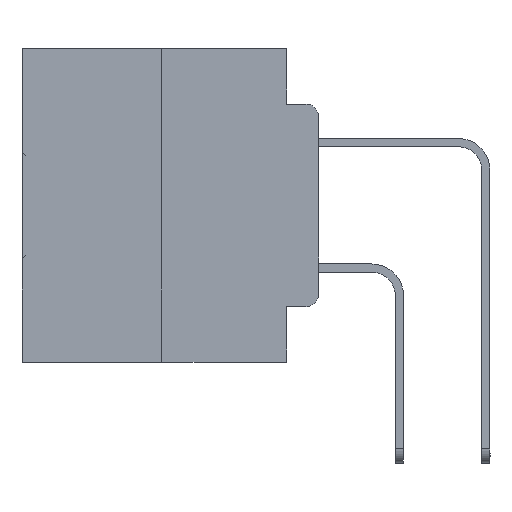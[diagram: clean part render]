
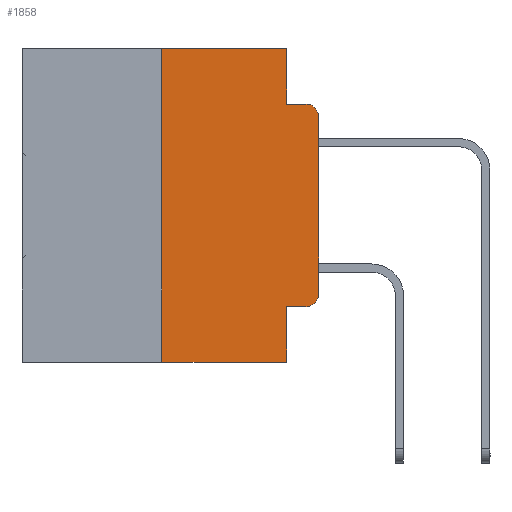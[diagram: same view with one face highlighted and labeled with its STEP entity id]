
A CAD part, left-side view. The second image highlights one B-rep face of the part: STEP entity #1858.
In plain terms, the highlighted planar face has unit normal (-1, 0, 0).
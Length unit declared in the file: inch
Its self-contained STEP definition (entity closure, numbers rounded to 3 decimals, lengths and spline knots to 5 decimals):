
#22 = CARTESIAN_POINT ( 'NONE',  ( 0., 0.25, 0. ) ) ;
#199 = ORIENTED_EDGE ( 'NONE', *, *, #5075, .F. ) ;
#231 = LINE ( 'NONE', #3575, #17360 ) ;
#294 = DIRECTION ( 'NONE',  ( -1., 0., 0. ) ) ;
#1390 = EDGE_CURVE ( 'NONE', #17032, #9484, #21260, .T. ) ;
#1604 = VECTOR ( 'NONE', #10682, 39.37008 ) ;
#1858 = ADVANCED_FACE ( 'NONE', ( #7118 ), #23116, .F. ) ;
#3144 = CARTESIAN_POINT ( 'NONE',  ( 0., 0., -0.3915 ) ) ;
#3575 = CARTESIAN_POINT ( 'NONE',  ( 0., 0., 0. ) ) ;
#3647 = AXIS2_PLACEMENT_3D ( 'NONE', #30141, #19464, #21884 ) ;
#4363 = VECTOR ( 'NONE', #18520, 39.37008 ) ;
#5075 = EDGE_CURVE ( 'NONE', #10746, #28352, #26570, .T. ) ;
#5642 = CARTESIAN_POINT ( 'NONE',  ( 0., 0.473, 0. ) ) ;
#6582 = CARTESIAN_POINT ( 'NONE',  ( 0., 0.051, -0.0885 ) ) ;
#6730 = CARTESIAN_POINT ( 'NONE',  ( 0., 0.473, 0. ) ) ;
#6943 = DIRECTION ( 'NONE',  ( 0., -1., 0. ) ) ;
#7118 = FACE_OUTER_BOUND ( 'NONE', #14256, .T. ) ;
#7145 = CARTESIAN_POINT ( 'NONE',  ( 0., 0.051, -0.5 ) ) ;
#8038 = CARTESIAN_POINT ( 'NONE',  ( 0., 0.051, 0. ) ) ;
#8712 = ORIENTED_EDGE ( 'NONE', *, *, #24335, .F. ) ;
#9397 = EDGE_CURVE ( 'NONE', #28352, #13922, #19731, .T. ) ;
#9484 = VERTEX_POINT ( 'NONE', #28569 ) ;
#10420 = CIRCLE ( 'NONE', #10743, 0.02 ) ;
#10559 = VECTOR ( 'NONE', #24782, 39.37008 ) ;
#10682 = DIRECTION ( 'NONE',  ( 0., 0., 1. ) ) ;
#10743 = AXIS2_PLACEMENT_3D ( 'NONE', #27555, #294, #19522 ) ;
#10746 = VERTEX_POINT ( 'NONE', #14887 ) ;
#10844 = CARTESIAN_POINT ( 'NONE',  ( 0., 0.25, -0.5 ) ) ;
#11346 = ORIENTED_EDGE ( 'NONE', *, *, #9397, .F. ) ;
#12129 = ORIENTED_EDGE ( 'NONE', *, *, #1390, .F. ) ;
#12223 = VECTOR ( 'NONE', #17129, 39.37008 ) ;
#13192 = ORIENTED_EDGE ( 'NONE', *, *, #17278, .T. ) ;
#13922 = VERTEX_POINT ( 'NONE', #33876 ) ;
#13999 = EDGE_CURVE ( 'NONE', #17032, #24507, #29745, .T. ) ;
#14052 = CARTESIAN_POINT ( 'NONE',  ( 0., 0.051, -0.4115 ) ) ;
#14256 = EDGE_LOOP ( 'NONE', ( #22071, #32693, #11346, #199, #30178, #12129, #21012, #8712, #13192, #14277 ) ) ;
#14277 = ORIENTED_EDGE ( 'NONE', *, *, #23934, .T. ) ;
#14463 = AXIS2_PLACEMENT_3D ( 'NONE', #6730, #34080, #25751 ) ;
#14887 = CARTESIAN_POINT ( 'NONE',  ( 0., 0.051, 0. ) ) ;
#15261 = CARTESIAN_POINT ( 'NONE',  ( 0., 0.051, 0. ) ) ;
#17032 = VERTEX_POINT ( 'NONE', #10844 ) ;
#17129 = DIRECTION ( 'NONE',  ( 0., -1., 0. ) ) ;
#17278 = EDGE_CURVE ( 'NONE', #30012, #27036, #19028, .T. ) ;
#17360 = VECTOR ( 'NONE', #19700, 39.37008 ) ;
#17816 = LINE ( 'NONE', #5642, #10559 ) ;
#18009 = DIRECTION ( 'NONE',  ( 0., 0., -1. ) ) ;
#18520 = DIRECTION ( 'NONE',  ( 0., 0., -1. ) ) ;
#18726 = CARTESIAN_POINT ( 'NONE',  ( 0., 0., -0.1085 ) ) ;
#19028 = LINE ( 'NONE', #33123, #12223 ) ;
#19464 = DIRECTION ( 'NONE',  ( -1., 0., 0. ) ) ;
#19522 = DIRECTION ( 'NONE',  ( 0., 0., -1. ) ) ;
#19700 = DIRECTION ( 'NONE',  ( 0., 0., 1. ) ) ;
#19731 = LINE ( 'NONE', #6582, #27869 ) ;
#20328 = VERTEX_POINT ( 'NONE', #3144 ) ;
#20470 = DIRECTION ( 'NONE',  ( 0., -1., 0. ) ) ;
#21012 = ORIENTED_EDGE ( 'NONE', *, *, #13999, .T. ) ;
#21260 = LINE ( 'NONE', #22, #1604 ) ;
#21812 = VERTEX_POINT ( 'NONE', #18726 ) ;
#21884 = DIRECTION ( 'NONE',  ( 0., 0., -1. ) ) ;
#22071 = ORIENTED_EDGE ( 'NONE', *, *, #25564, .T. ) ;
#23116 = PLANE ( 'NONE',  #14463 ) ;
#23934 = EDGE_CURVE ( 'NONE', #27036, #20328, #10420, .T. ) ;
#24072 = LINE ( 'NONE', #8038, #4363 ) ;
#24335 = EDGE_CURVE ( 'NONE', #30012, #24507, #24072, .T. ) ;
#24507 = VERTEX_POINT ( 'NONE', #7145 ) ;
#24561 = CARTESIAN_POINT ( 'NONE',  ( 0., 0.02, -0.4115 ) ) ;
#24620 = VECTOR ( 'NONE', #20470, 39.37008 ) ;
#24782 = DIRECTION ( 'NONE',  ( 0., -1., 0. ) ) ;
#25406 = EDGE_CURVE ( 'NONE', #21812, #13922, #31435, .T. ) ;
#25564 = EDGE_CURVE ( 'NONE', #20328, #21812, #231, .T. ) ;
#25751 = DIRECTION ( 'NONE',  ( 0., 0., -1. ) ) ;
#26570 = LINE ( 'NONE', #15261, #30386 ) ;
#27036 = VERTEX_POINT ( 'NONE', #24561 ) ;
#27555 = CARTESIAN_POINT ( 'NONE',  ( 0., 0.02, -0.3915 ) ) ;
#27869 = VECTOR ( 'NONE', #6943, 39.37008 ) ;
#28352 = VERTEX_POINT ( 'NONE', #30427 ) ;
#28512 = CARTESIAN_POINT ( 'NONE',  ( 0., 0.473, -0.5 ) ) ;
#28569 = CARTESIAN_POINT ( 'NONE',  ( 0., 0.25, 0. ) ) ;
#29745 = LINE ( 'NONE', #28512, #24620 ) ;
#30012 = VERTEX_POINT ( 'NONE', #14052 ) ;
#30141 = CARTESIAN_POINT ( 'NONE',  ( 0., 0.02, -0.1085 ) ) ;
#30178 = ORIENTED_EDGE ( 'NONE', *, *, #30509, .F. ) ;
#30386 = VECTOR ( 'NONE', #18009, 39.37008 ) ;
#30427 = CARTESIAN_POINT ( 'NONE',  ( 0., 0.051, -0.0885 ) ) ;
#30509 = EDGE_CURVE ( 'NONE', #9484, #10746, #17816, .T. ) ;
#31435 = CIRCLE ( 'NONE', #3647, 0.02 ) ;
#32693 = ORIENTED_EDGE ( 'NONE', *, *, #25406, .T. ) ;
#33123 = CARTESIAN_POINT ( 'NONE',  ( 0., 0.051, -0.4115 ) ) ;
#33876 = CARTESIAN_POINT ( 'NONE',  ( 0., 0.02, -0.0885 ) ) ;
#34080 = DIRECTION ( 'NONE',  ( 1., 0., 0. ) ) ;
